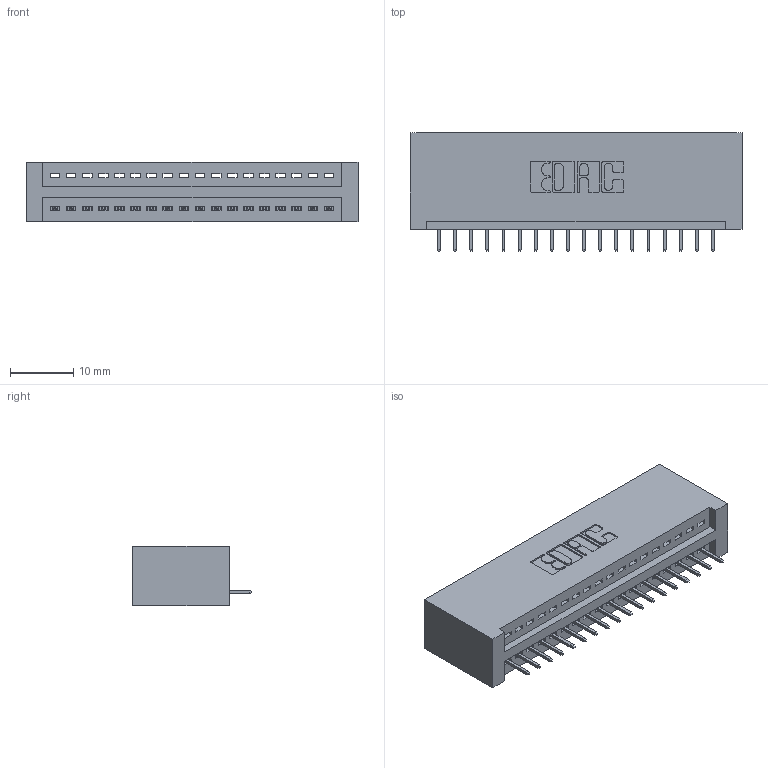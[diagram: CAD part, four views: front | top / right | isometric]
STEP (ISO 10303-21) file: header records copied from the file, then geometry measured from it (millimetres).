
FILE_DESCRIPTION (( 'STEP AP203' ), '1' );
FILE_NAME ('895-018-525-101.STEP', '2020-09-25T06:24:58', ( '' ), ( '' ), 'SwSTEP 2.0', 'SolidWorks 2020', '' );
FILE_SCHEMA (( 'CONFIG_CONTROL_DESIGN' ));
Length unit declared in the file: inch
Products named in the file (3): 845 Part_No Mounting Lugs; 345-292-001_345-293-125; 895-018-525-101
Assembly tree (19 placements, depth 2):
  895-018-525-101
    845 Part_No Mounting Lugs
    345-292-001_345-293-125  x18
Bounding box: 52.32 x 18.72 x 9.4 mm (x, y, z)
Volume: 5284.1 mm3; surface area: 6640.9 mm2
Topology: 19 solids, 19 shells, 1234 faces, 3557 edges, 2298 vertices
Faces by surface type: plane 904, cylinder 330
Entity records: 16575 total; most frequent: CARTESIAN_POINT 2878, ORIENTED_EDGE 2830, DIRECTION 2543, EDGE_CURVE 1415, VECTOR 1223, LINE 1223, VERTEX_POINT 938, AXIS2_PLACEMENT_3D 660
